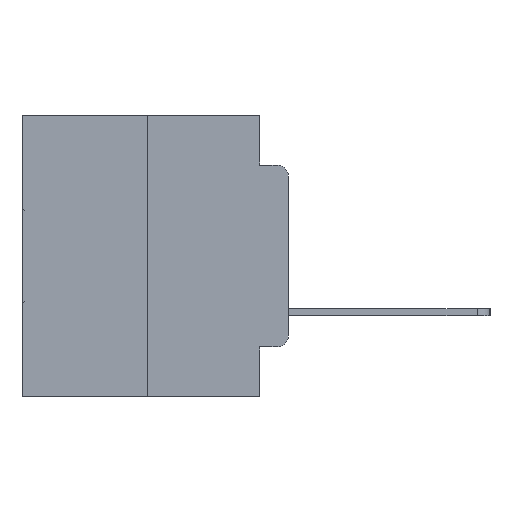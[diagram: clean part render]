
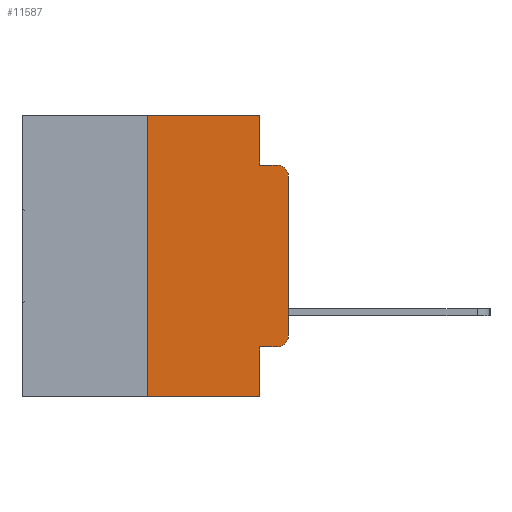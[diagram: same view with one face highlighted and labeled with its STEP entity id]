
A CAD part, left-side view. The second image highlights one B-rep face of the part: STEP entity #11587.
In plain terms, the highlighted planar face has unit normal (-1, 0, 0).
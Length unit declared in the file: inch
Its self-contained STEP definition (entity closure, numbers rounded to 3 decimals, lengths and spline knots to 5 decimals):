
#250 = EDGE_CURVE ( 'NONE', #5668, #29282, #6573, .T. ) ;
#384 = DIRECTION ( 'NONE',  ( 0., 0., -1. ) ) ;
#495 = VECTOR ( 'NONE', #28246, 39.37008 ) ;
#1257 = DIRECTION ( 'NONE',  ( 0., -1., 0. ) ) ;
#1357 = VECTOR ( 'NONE', #24385, 39.37008 ) ;
#2096 = VECTOR ( 'NONE', #1257, 39.37008 ) ;
#2440 = CARTESIAN_POINT ( 'NONE',  ( 0., 0.25, 0. ) ) ;
#2500 = ORIENTED_EDGE ( 'NONE', *, *, #30736, .F. ) ;
#4437 = VERTEX_POINT ( 'NONE', #25640 ) ;
#4695 = VECTOR ( 'NONE', #384, 39.37008 ) ;
#5237 = EDGE_CURVE ( 'NONE', #4437, #5668, #8139, .T. ) ;
#5668 = VERTEX_POINT ( 'NONE', #30747 ) ;
#5835 = CARTESIAN_POINT ( 'NONE',  ( 0., 0.051, -0.4115 ) ) ;
#6547 = VERTEX_POINT ( 'NONE', #22404 ) ;
#6573 = CIRCLE ( 'NONE', #11076, 0.02 ) ;
#6769 = ORIENTED_EDGE ( 'NONE', *, *, #14344, .T. ) ;
#7120 = LINE ( 'NONE', #30673, #495 ) ;
#7370 = EDGE_CURVE ( 'NONE', #6547, #18431, #28454, .T. ) ;
#7377 = AXIS2_PLACEMENT_3D ( 'NONE', #23040, #8185, #25529 ) ;
#7991 = LINE ( 'NONE', #21913, #1357 ) ;
#8139 = LINE ( 'NONE', #21824, #20602 ) ;
#8185 = DIRECTION ( 'NONE',  ( -1., 0., 0. ) ) ;
#8637 = VERTEX_POINT ( 'NONE', #5835 ) ;
#9487 = VECTOR ( 'NONE', #27386, 39.37008 ) ;
#9925 = VECTOR ( 'NONE', #30223, 39.37008 ) ;
#10676 = CARTESIAN_POINT ( 'NONE',  ( 0., 0.051, -0.5 ) ) ;
#11076 = AXIS2_PLACEMENT_3D ( 'NONE', #16176, #15004, #14890 ) ;
#11147 = CARTESIAN_POINT ( 'NONE',  ( 0., 0.051, -0.0885 ) ) ;
#11496 = LINE ( 'NONE', #15482, #9925 ) ;
#11587 = ADVANCED_FACE ( 'NONE', ( #26797 ), #11886, .F. ) ;
#11860 = VECTOR ( 'NONE', #15247, 39.37008 ) ;
#11886 = PLANE ( 'NONE',  #23582 ) ;
#12170 = LINE ( 'NONE', #30043, #4695 ) ;
#13209 = ORIENTED_EDGE ( 'NONE', *, *, #250, .T. ) ;
#13492 = ORIENTED_EDGE ( 'NONE', *, *, #27476, .F. ) ;
#14344 = EDGE_CURVE ( 'NONE', #19101, #4437, #20878, .T. ) ;
#14355 = CARTESIAN_POINT ( 'NONE',  ( 0., 0.473, 0. ) ) ;
#14464 = DIRECTION ( 'NONE',  ( 0., 0., -1. ) ) ;
#14521 = DIRECTION ( 'NONE',  ( 0., 0., 1. ) ) ;
#14890 = DIRECTION ( 'NONE',  ( 0., 0., -1. ) ) ;
#15004 = DIRECTION ( 'NONE',  ( -1., 0., 0. ) ) ;
#15247 = DIRECTION ( 'NONE',  ( 0., -1., 0. ) ) ;
#15482 = CARTESIAN_POINT ( 'NONE',  ( 0., 0.051, -0.0885 ) ) ;
#16009 = EDGE_CURVE ( 'NONE', #8637, #19101, #18532, .T. ) ;
#16176 = CARTESIAN_POINT ( 'NONE',  ( 0., 0.02, -0.1085 ) ) ;
#17639 = EDGE_CURVE ( 'NONE', #8637, #18431, #7991, .T. ) ;
#18316 = CARTESIAN_POINT ( 'NONE',  ( 0., 0.02, -0.4115 ) ) ;
#18431 = VERTEX_POINT ( 'NONE', #10676 ) ;
#18532 = LINE ( 'NONE', #29879, #11860 ) ;
#18882 = EDGE_LOOP ( 'NONE', ( #19381, #13209, #2500, #19239, #22506, #13492, #25968, #26571, #28707, #6769 ) ) ;
#18934 = EDGE_CURVE ( 'NONE', #24299, #31192, #22642, .T. ) ;
#19101 = VERTEX_POINT ( 'NONE', #18316 ) ;
#19239 = ORIENTED_EDGE ( 'NONE', *, *, #29107, .F. ) ;
#19381 = ORIENTED_EDGE ( 'NONE', *, *, #5237, .T. ) ;
#20295 = CARTESIAN_POINT ( 'NONE',  ( 0., 0.051, 0. ) ) ;
#20602 = VECTOR ( 'NONE', #14521, 39.37008 ) ;
#20878 = CIRCLE ( 'NONE', #7377, 0.02 ) ;
#21824 = CARTESIAN_POINT ( 'NONE',  ( 0., 0., 0. ) ) ;
#21913 = CARTESIAN_POINT ( 'NONE',  ( 0., 0.051, 0. ) ) ;
#22404 = CARTESIAN_POINT ( 'NONE',  ( 0., 0.25, -0.5 ) ) ;
#22506 = ORIENTED_EDGE ( 'NONE', *, *, #18934, .F. ) ;
#22642 = LINE ( 'NONE', #24943, #9487 ) ;
#23040 = CARTESIAN_POINT ( 'NONE',  ( 0., 0.02, -0.3915 ) ) ;
#23582 = AXIS2_PLACEMENT_3D ( 'NONE', #14355, #29121, #14464 ) ;
#23611 = VERTEX_POINT ( 'NONE', #11147 ) ;
#24299 = VERTEX_POINT ( 'NONE', #2440 ) ;
#24385 = DIRECTION ( 'NONE',  ( 0., 0., -1. ) ) ;
#24943 = CARTESIAN_POINT ( 'NONE',  ( 0., 0.473, 0. ) ) ;
#25529 = DIRECTION ( 'NONE',  ( 0., 0., -1. ) ) ;
#25640 = CARTESIAN_POINT ( 'NONE',  ( 0., 0., -0.3915 ) ) ;
#25924 = CARTESIAN_POINT ( 'NONE',  ( 0., 0.02, -0.0885 ) ) ;
#25968 = ORIENTED_EDGE ( 'NONE', *, *, #7370, .T. ) ;
#26571 = ORIENTED_EDGE ( 'NONE', *, *, #17639, .F. ) ;
#26797 = FACE_OUTER_BOUND ( 'NONE', #18882, .T. ) ;
#27386 = DIRECTION ( 'NONE',  ( 0., -1., 0. ) ) ;
#27476 = EDGE_CURVE ( 'NONE', #6547, #24299, #7120, .T. ) ;
#28246 = DIRECTION ( 'NONE',  ( 0., 0., 1. ) ) ;
#28452 = CARTESIAN_POINT ( 'NONE',  ( 0., 0.473, -0.5 ) ) ;
#28454 = LINE ( 'NONE', #28452, #2096 ) ;
#28707 = ORIENTED_EDGE ( 'NONE', *, *, #16009, .T. ) ;
#29107 = EDGE_CURVE ( 'NONE', #31192, #23611, #12170, .T. ) ;
#29121 = DIRECTION ( 'NONE',  ( 1., 0., 0. ) ) ;
#29282 = VERTEX_POINT ( 'NONE', #25924 ) ;
#29879 = CARTESIAN_POINT ( 'NONE',  ( 0., 0.051, -0.4115 ) ) ;
#30043 = CARTESIAN_POINT ( 'NONE',  ( 0., 0.051, 0. ) ) ;
#30223 = DIRECTION ( 'NONE',  ( 0., -1., 0. ) ) ;
#30673 = CARTESIAN_POINT ( 'NONE',  ( 0., 0.25, 0. ) ) ;
#30736 = EDGE_CURVE ( 'NONE', #23611, #29282, #11496, .T. ) ;
#30747 = CARTESIAN_POINT ( 'NONE',  ( 0., 0., -0.1085 ) ) ;
#31192 = VERTEX_POINT ( 'NONE', #20295 ) ;
